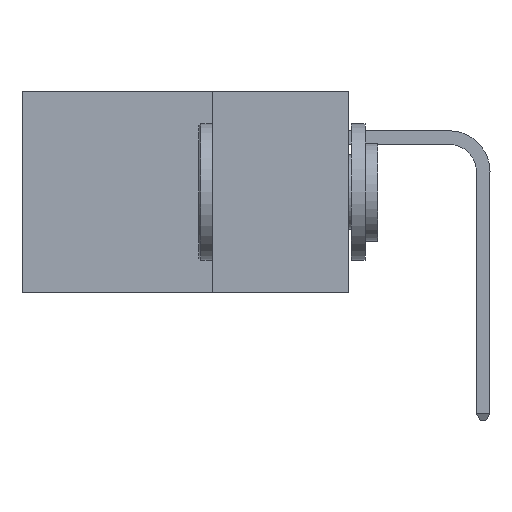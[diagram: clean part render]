
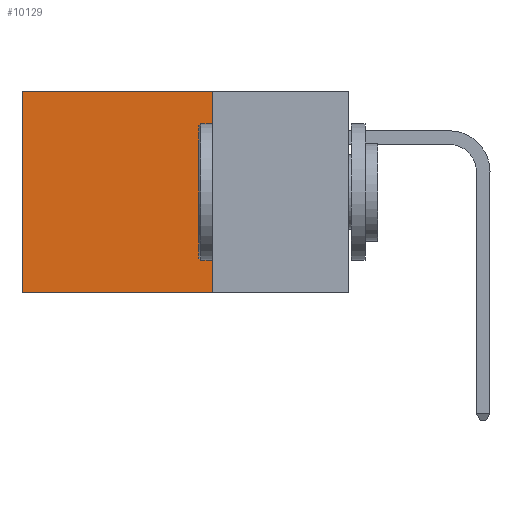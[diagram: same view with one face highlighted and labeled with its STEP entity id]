
A CAD part, left-side view. The second image highlights one B-rep face of the part: STEP entity #10129.
In plain terms, the highlighted planar face has unit normal (-1, 0, 0).
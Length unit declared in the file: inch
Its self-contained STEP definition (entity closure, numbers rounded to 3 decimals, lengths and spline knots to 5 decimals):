
#229 = DIRECTION ( 'NONE',  ( 0., 0., -1. ) ) ;
#619 = EDGE_CURVE ( 'NONE', #11013, #17272, #17020, .T. ) ;
#1642 = DIRECTION ( 'NONE',  ( 0., 0., -1. ) ) ;
#2378 = ORIENTED_EDGE ( 'NONE', *, *, #25488, .T. ) ;
#2822 = ORIENTED_EDGE ( 'NONE', *, *, #15146, .F. ) ;
#3260 = PLANE ( 'NONE',  #16997 ) ;
#3635 = ORIENTED_EDGE ( 'NONE', *, *, #619, .F. ) ;
#4120 = LINE ( 'NONE', #12099, #24773 ) ;
#5386 = DIRECTION ( 'NONE',  ( 0., 0., -1. ) ) ;
#5550 = VECTOR ( 'NONE', #20102, 39.37008 ) ;
#5983 = CARTESIAN_POINT ( 'NONE',  ( 0.2875, 0.25, -0.37 ) ) ;
#8076 = LINE ( 'NONE', #8555, #23851 ) ;
#8555 = CARTESIAN_POINT ( 'NONE',  ( 0.2875, 0.25, 0. ) ) ;
#8689 = CARTESIAN_POINT ( 'NONE',  ( 0.2875, 0.25, 0. ) ) ;
#9052 = EDGE_CURVE ( 'NONE', #18912, #9407, #21411, .T. ) ;
#9407 = VERTEX_POINT ( 'NONE', #25306 ) ;
#9771 = CARTESIAN_POINT ( 'NONE',  ( 0.2875, 0.25, 0. ) ) ;
#10129 = ADVANCED_FACE ( 'NONE', ( #15538 ), #3260, .F. ) ;
#10544 = CARTESIAN_POINT ( 'NONE',  ( 0.2875, 0.25, -0.37 ) ) ;
#11013 = VERTEX_POINT ( 'NONE', #5983 ) ;
#11492 = VECTOR ( 'NONE', #22945, 39.37008 ) ;
#11707 = ORIENTED_EDGE ( 'NONE', *, *, #9052, .T. ) ;
#12099 = CARTESIAN_POINT ( 'NONE',  ( 0.2875, 0.6, 0. ) ) ;
#15146 = EDGE_CURVE ( 'NONE', #18912, #11013, #8076, .T. ) ;
#15538 = FACE_OUTER_BOUND ( 'NONE', #18279, .T. ) ;
#15704 = CARTESIAN_POINT ( 'NONE',  ( 0.2875, 0.25, 0. ) ) ;
#16997 = AXIS2_PLACEMENT_3D ( 'NONE', #15704, #17823, #5386 ) ;
#17020 = LINE ( 'NONE', #10544, #11492 ) ;
#17272 = VERTEX_POINT ( 'NONE', #21455 ) ;
#17823 = DIRECTION ( 'NONE',  ( 1., 0., 0. ) ) ;
#18279 = EDGE_LOOP ( 'NONE', ( #2378, #3635, #2822, #11707 ) ) ;
#18912 = VERTEX_POINT ( 'NONE', #8689 ) ;
#20102 = DIRECTION ( 'NONE',  ( 0., 1., 0. ) ) ;
#21411 = LINE ( 'NONE', #9771, #5550 ) ;
#21455 = CARTESIAN_POINT ( 'NONE',  ( 0.2875, 0.6, -0.37 ) ) ;
#22945 = DIRECTION ( 'NONE',  ( 0., 1., 0. ) ) ;
#23851 = VECTOR ( 'NONE', #229, 39.37008 ) ;
#24773 = VECTOR ( 'NONE', #1642, 39.37008 ) ;
#25306 = CARTESIAN_POINT ( 'NONE',  ( 0.2875, 0.6, 0. ) ) ;
#25488 = EDGE_CURVE ( 'NONE', #9407, #17272, #4120, .T. ) ;
